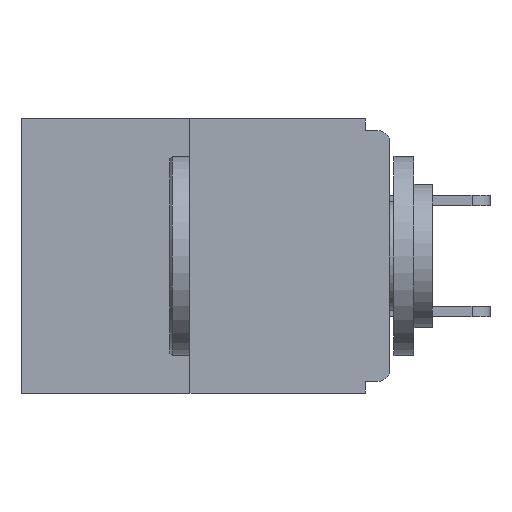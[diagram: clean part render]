
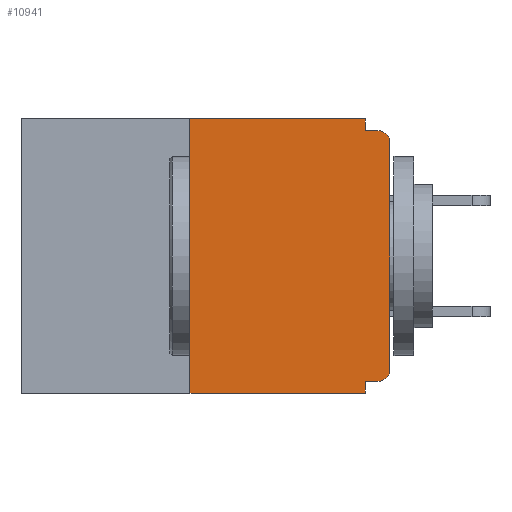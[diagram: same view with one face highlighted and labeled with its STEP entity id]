
A CAD part, left-side view. The second image highlights one B-rep face of the part: STEP entity #10941.
In plain terms, the highlighted planar face has unit normal (-1, 0, 0).
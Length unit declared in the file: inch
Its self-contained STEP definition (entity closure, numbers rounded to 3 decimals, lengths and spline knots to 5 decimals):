
#358 = VERTEX_POINT ( 'NONE', #18270 ) ;
#541 = CARTESIAN_POINT ( 'NONE',  ( 0., 0.031, -0.343 ) ) ;
#696 = CARTESIAN_POINT ( 'NONE',  ( 0., 0.031, -0.328 ) ) ;
#824 = EDGE_CURVE ( 'NONE', #11642, #13340, #7104, .T. ) ;
#863 = EDGE_LOOP ( 'NONE', ( #17267, #18995, #7846, #17182, #9530, #15431, #11396, #15587, #7901, #11471 ) ) ;
#1074 = VECTOR ( 'NONE', #2249, 39.37008 ) ;
#1199 = LINE ( 'NONE', #7899, #8084 ) ;
#1326 = EDGE_CURVE ( 'NONE', #12188, #358, #8973, .T. ) ;
#1791 = DIRECTION ( 'NONE',  ( 0., 0., -1. ) ) ;
#2125 = CARTESIAN_POINT ( 'NONE',  ( 0., 0.25, 0. ) ) ;
#2232 = VERTEX_POINT ( 'NONE', #3453 ) ;
#2249 = DIRECTION ( 'NONE',  ( 0., 0., 1. ) ) ;
#3126 = DIRECTION ( 'NONE',  ( -1., 0., 0. ) ) ;
#3453 = CARTESIAN_POINT ( 'NONE',  ( 0., 0.25, 0. ) ) ;
#3900 = AXIS2_PLACEMENT_3D ( 'NONE', #4305, #6102, #16538 ) ;
#4157 = CARTESIAN_POINT ( 'NONE',  ( 0., 0.015, -0.328 ) ) ;
#4305 = CARTESIAN_POINT ( 'NONE',  ( 0., 0.015, -0.03 ) ) ;
#4548 = CARTESIAN_POINT ( 'NONE',  ( 0., 0.46, 0. ) ) ;
#4586 = DIRECTION ( 'NONE',  ( 0., 0., -1. ) ) ;
#4711 = VERTEX_POINT ( 'NONE', #6650 ) ;
#4804 = VECTOR ( 'NONE', #16423, 39.37008 ) ;
#5082 = AXIS2_PLACEMENT_3D ( 'NONE', #4548, #16581, #19383 ) ;
#5663 = EDGE_CURVE ( 'NONE', #13990, #4711, #5701, .T. ) ;
#5701 = CIRCLE ( 'NONE', #6270, 0.015 ) ;
#6078 = PLANE ( 'NONE',  #5082 ) ;
#6102 = DIRECTION ( 'NONE',  ( -1., 0., 0. ) ) ;
#6270 = AXIS2_PLACEMENT_3D ( 'NONE', #11936, #3126, #4586 ) ;
#6650 = CARTESIAN_POINT ( 'NONE',  ( 0., 0., -0.313 ) ) ;
#6821 = EDGE_CURVE ( 'NONE', #4711, #12188, #14963, .T. ) ;
#7104 = LINE ( 'NONE', #541, #16047 ) ;
#7521 = DIRECTION ( 'NONE',  ( 0., 1., 0. ) ) ;
#7736 = CARTESIAN_POINT ( 'NONE',  ( 0., 0.25, -0.343 ) ) ;
#7755 = EDGE_CURVE ( 'NONE', #2232, #11207, #1199, .T. ) ;
#7846 = ORIENTED_EDGE ( 'NONE', *, *, #10204, .T. ) ;
#7899 = CARTESIAN_POINT ( 'NONE',  ( 0., 0.46, 0. ) ) ;
#7901 = ORIENTED_EDGE ( 'NONE', *, *, #18559, .F. ) ;
#7912 = DIRECTION ( 'NONE',  ( 0., 0., 1. ) ) ;
#8084 = VECTOR ( 'NONE', #12460, 39.37008 ) ;
#8237 = VECTOR ( 'NONE', #9103, 39.37008 ) ;
#8665 = LINE ( 'NONE', #2125, #1074 ) ;
#8926 = CARTESIAN_POINT ( 'NONE',  ( 0., 0.031, 0. ) ) ;
#8973 = CIRCLE ( 'NONE', #3900, 0.015 ) ;
#9103 = DIRECTION ( 'NONE',  ( 0., -1., 0. ) ) ;
#9264 = VERTEX_POINT ( 'NONE', #7736 ) ;
#9530 = ORIENTED_EDGE ( 'NONE', *, *, #18471, .F. ) ;
#9615 = VERTEX_POINT ( 'NONE', #12550 ) ;
#9658 = LINE ( 'NONE', #13704, #8237 ) ;
#10086 = LINE ( 'NONE', #11096, #18564 ) ;
#10204 = EDGE_CURVE ( 'NONE', #9264, #13340, #9658, .T. ) ;
#10941 = ADVANCED_FACE ( 'NONE', ( #15725 ), #6078, .F. ) ;
#11096 = CARTESIAN_POINT ( 'NONE',  ( 0., 0., -0.015 ) ) ;
#11207 = VERTEX_POINT ( 'NONE', #15875 ) ;
#11396 = ORIENTED_EDGE ( 'NONE', *, *, #6821, .T. ) ;
#11471 = ORIENTED_EDGE ( 'NONE', *, *, #12513, .F. ) ;
#11642 = VERTEX_POINT ( 'NONE', #696 ) ;
#11936 = CARTESIAN_POINT ( 'NONE',  ( 0., 0.015, -0.313 ) ) ;
#12188 = VERTEX_POINT ( 'NONE', #18476 ) ;
#12225 = VECTOR ( 'NONE', #7521, 39.37008 ) ;
#12460 = DIRECTION ( 'NONE',  ( 0., -1., 0. ) ) ;
#12513 = EDGE_CURVE ( 'NONE', #11207, #9615, #13331, .T. ) ;
#12550 = CARTESIAN_POINT ( 'NONE',  ( 0., 0.031, -0.015 ) ) ;
#13086 = VECTOR ( 'NONE', #7912, 39.37008 ) ;
#13331 = LINE ( 'NONE', #8926, #4804 ) ;
#13340 = VERTEX_POINT ( 'NONE', #13645 ) ;
#13606 = CARTESIAN_POINT ( 'NONE',  ( 0., 0., -0.328 ) ) ;
#13645 = CARTESIAN_POINT ( 'NONE',  ( 0., 0.031, -0.343 ) ) ;
#13704 = CARTESIAN_POINT ( 'NONE',  ( 0., 0.46, -0.343 ) ) ;
#13990 = VERTEX_POINT ( 'NONE', #4157 ) ;
#14963 = LINE ( 'NONE', #16756, #13086 ) ;
#15431 = ORIENTED_EDGE ( 'NONE', *, *, #5663, .T. ) ;
#15587 = ORIENTED_EDGE ( 'NONE', *, *, #1326, .T. ) ;
#15725 = FACE_OUTER_BOUND ( 'NONE', #863, .T. ) ;
#15875 = CARTESIAN_POINT ( 'NONE',  ( 0., 0.031, 0. ) ) ;
#16047 = VECTOR ( 'NONE', #1791, 39.37008 ) ;
#16226 = LINE ( 'NONE', #13606, #12225 ) ;
#16423 = DIRECTION ( 'NONE',  ( 0., 0., -1. ) ) ;
#16538 = DIRECTION ( 'NONE',  ( 0., 0., -1. ) ) ;
#16581 = DIRECTION ( 'NONE',  ( 1., 0., 0. ) ) ;
#16756 = CARTESIAN_POINT ( 'NONE',  ( 0., 0., 0. ) ) ;
#17168 = DIRECTION ( 'NONE',  ( 0., -1., 0. ) ) ;
#17182 = ORIENTED_EDGE ( 'NONE', *, *, #824, .F. ) ;
#17267 = ORIENTED_EDGE ( 'NONE', *, *, #7755, .F. ) ;
#17997 = EDGE_CURVE ( 'NONE', #9264, #2232, #8665, .T. ) ;
#18270 = CARTESIAN_POINT ( 'NONE',  ( 0., 0.015, -0.015 ) ) ;
#18471 = EDGE_CURVE ( 'NONE', #13990, #11642, #16226, .T. ) ;
#18476 = CARTESIAN_POINT ( 'NONE',  ( 0., 0., -0.03 ) ) ;
#18559 = EDGE_CURVE ( 'NONE', #9615, #358, #10086, .T. ) ;
#18564 = VECTOR ( 'NONE', #17168, 39.37008 ) ;
#18995 = ORIENTED_EDGE ( 'NONE', *, *, #17997, .F. ) ;
#19383 = DIRECTION ( 'NONE',  ( 0., 0., -1. ) ) ;
